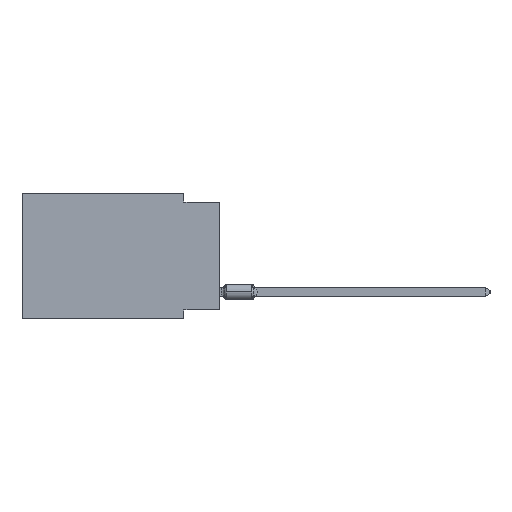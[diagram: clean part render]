
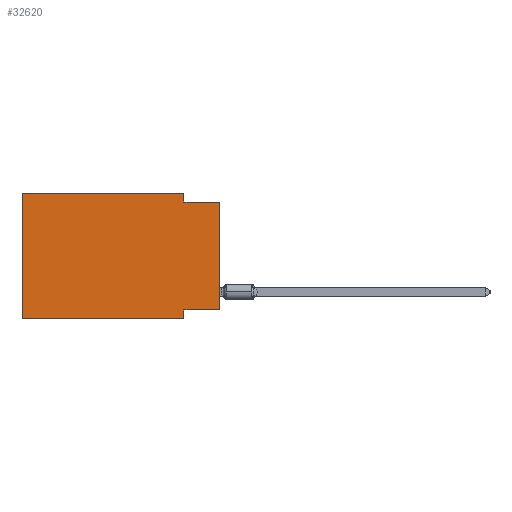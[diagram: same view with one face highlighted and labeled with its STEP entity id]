
A CAD part, left-side view. The second image highlights one B-rep face of the part: STEP entity #32620.
In plain terms, the highlighted planar face has unit normal (-1, 0, 0).
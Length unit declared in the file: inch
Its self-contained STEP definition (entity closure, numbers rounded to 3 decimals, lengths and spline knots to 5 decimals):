
#1723 = DIRECTION ( 'NONE',  ( 0., -1., 0. ) ) ;
#1843 = DIRECTION ( 'NONE',  ( 0., -1., 0. ) ) ;
#1893 = VERTEX_POINT ( 'NONE', #46122 ) ;
#2058 = ORIENTED_EDGE ( 'NONE', *, *, #8818, .F. ) ;
#2789 = DIRECTION ( 'NONE',  ( 0., 0., 1. ) ) ;
#3714 = EDGE_CURVE ( 'NONE', #46439, #31405, #20261, .T. ) ;
#4859 = CARTESIAN_POINT ( 'NONE',  ( 0., 0., -0.025 ) ) ;
#4955 = LINE ( 'NONE', #13706, #51564 ) ;
#5072 = VECTOR ( 'NONE', #1843, 39.37008 ) ;
#5449 = ORIENTED_EDGE ( 'NONE', *, *, #34131, .F. ) ;
#6422 = EDGE_CURVE ( 'NONE', #1893, #18057, #9784, .T. ) ;
#6877 = VECTOR ( 'NONE', #18106, 39.37008 ) ;
#8818 = EDGE_CURVE ( 'NONE', #52979, #31405, #21680, .T. ) ;
#9784 = LINE ( 'NONE', #47608, #5072 ) ;
#9874 = CARTESIAN_POINT ( 'NONE',  ( 0., 0.1, -0.35 ) ) ;
#10443 = VECTOR ( 'NONE', #1723, 39.37008 ) ;
#10582 = LINE ( 'NONE', #23473, #27212 ) ;
#11811 = CARTESIAN_POINT ( 'NONE',  ( 0., 0.1, -0.025 ) ) ;
#13706 = CARTESIAN_POINT ( 'NONE',  ( 0., 0., 0. ) ) ;
#14163 = DIRECTION ( 'NONE',  ( 0., 1., 0. ) ) ;
#15280 = CARTESIAN_POINT ( 'NONE',  ( 0., 0.1, -0.325 ) ) ;
#15484 = ORIENTED_EDGE ( 'NONE', *, *, #34373, .F. ) ;
#16195 = EDGE_CURVE ( 'NONE', #25389, #34030, #22285, .T. ) ;
#16316 = DIRECTION ( 'NONE',  ( 1., 0., 0. ) ) ;
#16710 = EDGE_CURVE ( 'NONE', #48045, #34030, #4955, .T. ) ;
#18057 = VERTEX_POINT ( 'NONE', #40271 ) ;
#18106 = DIRECTION ( 'NONE',  ( 0., 0., -1. ) ) ;
#18373 = DIRECTION ( 'NONE',  ( 0., 0., 1. ) ) ;
#18564 = CARTESIAN_POINT ( 'NONE',  ( 0., 0.1, -0.35 ) ) ;
#20261 = LINE ( 'NONE', #53141, #35253 ) ;
#21680 = LINE ( 'NONE', #9874, #6877 ) ;
#22285 = LINE ( 'NONE', #39569, #10443 ) ;
#23473 = CARTESIAN_POINT ( 'NONE',  ( 0., 0., -0.325 ) ) ;
#23525 = CARTESIAN_POINT ( 'NONE',  ( 0., 0.55, -0.35 ) ) ;
#24450 = AXIS2_PLACEMENT_3D ( 'NONE', #24824, #16316, #54122 ) ;
#24824 = CARTESIAN_POINT ( 'NONE',  ( 0., 0.55, 0. ) ) ;
#24831 = LINE ( 'NONE', #48945, #39485 ) ;
#25389 = VERTEX_POINT ( 'NONE', #11811 ) ;
#27212 = VECTOR ( 'NONE', #14163, 39.37008 ) ;
#28068 = ORIENTED_EDGE ( 'NONE', *, *, #36766, .F. ) ;
#28114 = DIRECTION ( 'NONE',  ( 0., 0., -1. ) ) ;
#29198 = PLANE ( 'NONE',  #24450 ) ;
#31405 = VERTEX_POINT ( 'NONE', #18564 ) ;
#32620 = ADVANCED_FACE ( 'NONE', ( #50812 ), #29198, .F. ) ;
#34030 = VERTEX_POINT ( 'NONE', #4859 ) ;
#34131 = EDGE_CURVE ( 'NONE', #48045, #52979, #10582, .T. ) ;
#34373 = EDGE_CURVE ( 'NONE', #18057, #25389, #24831, .T. ) ;
#34662 = ORIENTED_EDGE ( 'NONE', *, *, #6422, .F. ) ;
#34718 = EDGE_LOOP ( 'NONE', ( #43414, #51980, #15484, #34662, #28068, #52499, #2058, #5449 ) ) ;
#35253 = VECTOR ( 'NONE', #44661, 39.37008 ) ;
#36766 = EDGE_CURVE ( 'NONE', #46439, #1893, #40645, .T. ) ;
#39485 = VECTOR ( 'NONE', #28114, 39.37008 ) ;
#39569 = CARTESIAN_POINT ( 'NONE',  ( 0., 0., -0.025 ) ) ;
#40271 = CARTESIAN_POINT ( 'NONE',  ( 0., 0.1, 0. ) ) ;
#40645 = LINE ( 'NONE', #52108, #47513 ) ;
#43414 = ORIENTED_EDGE ( 'NONE', *, *, #16710, .T. ) ;
#44661 = DIRECTION ( 'NONE',  ( 0., -1., 0. ) ) ;
#46122 = CARTESIAN_POINT ( 'NONE',  ( 0., 0.55, 0. ) ) ;
#46439 = VERTEX_POINT ( 'NONE', #23525 ) ;
#47513 = VECTOR ( 'NONE', #2789, 39.37008 ) ;
#47608 = CARTESIAN_POINT ( 'NONE',  ( 0., 0.55, 0. ) ) ;
#47844 = CARTESIAN_POINT ( 'NONE',  ( 0., 0., -0.325 ) ) ;
#48045 = VERTEX_POINT ( 'NONE', #47844 ) ;
#48945 = CARTESIAN_POINT ( 'NONE',  ( 0., 0.1, 0. ) ) ;
#50812 = FACE_OUTER_BOUND ( 'NONE', #34718, .T. ) ;
#51564 = VECTOR ( 'NONE', #18373, 39.37008 ) ;
#51980 = ORIENTED_EDGE ( 'NONE', *, *, #16195, .F. ) ;
#52108 = CARTESIAN_POINT ( 'NONE',  ( 0., 0.55, 0. ) ) ;
#52499 = ORIENTED_EDGE ( 'NONE', *, *, #3714, .T. ) ;
#52979 = VERTEX_POINT ( 'NONE', #15280 ) ;
#53141 = CARTESIAN_POINT ( 'NONE',  ( 0., 0.55, -0.35 ) ) ;
#54122 = DIRECTION ( 'NONE',  ( 0., 0., -1. ) ) ;
